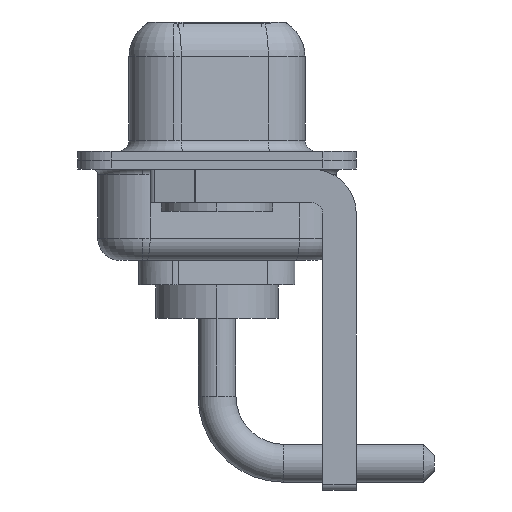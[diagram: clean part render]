
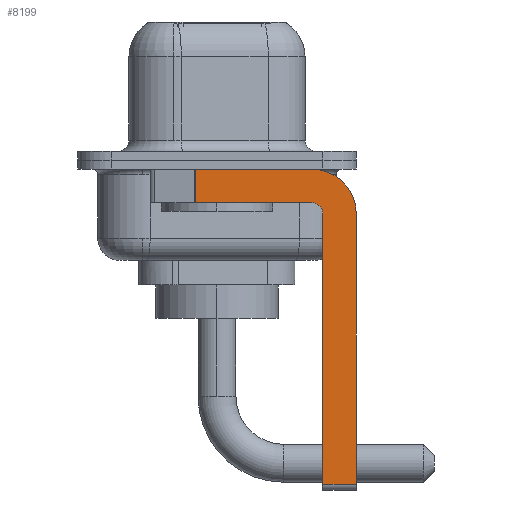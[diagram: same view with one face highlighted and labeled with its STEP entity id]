
A CAD part, left-side view. The second image highlights one B-rep face of the part: STEP entity #8199.
In plain terms, the highlighted planar face has unit normal (-1, 0, 0).
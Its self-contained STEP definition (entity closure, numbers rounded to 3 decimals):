
#23 = CARTESIAN_POINT ( 'NONE',  ( -2.9, -4.25, -2.4 ) ) ;
#88 = EDGE_CURVE ( 'NONE', #8358, #3053, #6449, .T. ) ;
#173 = VECTOR ( 'NONE', #2546, 1000. ) ;
#366 = AXIS2_PLACEMENT_3D ( 'NONE', #23, #11373, #2011 ) ;
#409 = CIRCLE ( 'NONE', #2136, 2. ) ;
#891 = CARTESIAN_POINT ( 'NONE',  ( -2.9, -4.25, -1.9 ) ) ;
#1414 = ORIENTED_EDGE ( 'NONE', *, *, #10089, .F. ) ;
#1885 = PLANE ( 'NONE',  #10585 ) ;
#2011 = DIRECTION ( 'NONE',  ( 0., 0., 1. ) ) ;
#2014 = DIRECTION ( 'NONE',  ( 0., 0., -1. ) ) ;
#2136 = AXIS2_PLACEMENT_3D ( 'NONE', #3379, #11724, #5716 ) ;
#2546 = DIRECTION ( 'NONE',  ( 0., 0., 1. ) ) ;
#2750 = VECTOR ( 'NONE', #5002, 1000. ) ;
#3053 = VERTEX_POINT ( 'NONE', #6929 ) ;
#3113 = CARTESIAN_POINT ( 'NONE',  ( -2.9, 0.978, -1.9 ) ) ;
#3173 = EDGE_CURVE ( 'NONE', #9849, #12831, #9085, .T. ) ;
#3239 = CARTESIAN_POINT ( 'NONE',  ( -2.9, -4.75, -14.55 ) ) ;
#3241 = CARTESIAN_POINT ( 'NONE',  ( -2.9, -4.75, -2.4 ) ) ;
#3379 = CARTESIAN_POINT ( 'NONE',  ( -2.9, -4.25, -2.4 ) ) ;
#3424 = EDGE_CURVE ( 'NONE', #8645, #9142, #409, .T. ) ;
#3811 = VECTOR ( 'NONE', #5895, 1000. ) ;
#4056 = EDGE_CURVE ( 'NONE', #10134, #8645, #8183, .T. ) ;
#4769 = DIRECTION ( 'NONE',  ( 0., 1., 0. ) ) ;
#4786 = EDGE_CURVE ( 'NONE', #12831, #7697, #13028, .T. ) ;
#4844 = ORIENTED_EDGE ( 'NONE', *, *, #5857, .T. ) ;
#5002 = DIRECTION ( 'NONE',  ( 0., -1., 0. ) ) ;
#5039 = FACE_OUTER_BOUND ( 'NONE', #12159, .T. ) ;
#5440 = DIRECTION ( 'NONE',  ( 0., -1., 0. ) ) ;
#5539 = ORIENTED_EDGE ( 'NONE', *, *, #88, .T. ) ;
#5698 = LINE ( 'NONE', #9858, #3811 ) ;
#5716 = DIRECTION ( 'NONE',  ( 0., 0., -1. ) ) ;
#5857 = EDGE_CURVE ( 'NONE', #10134, #7697, #5698, .T. ) ;
#5867 = ORIENTED_EDGE ( 'NONE', *, *, #3173, .F. ) ;
#5895 = DIRECTION ( 'NONE',  ( 0., 0., -1. ) ) ;
#6449 = LINE ( 'NONE', #10602, #9518 ) ;
#6718 = ORIENTED_EDGE ( 'NONE', *, *, #4056, .F. ) ;
#6838 = VECTOR ( 'NONE', #4769, 1000. ) ;
#6929 = CARTESIAN_POINT ( 'NONE',  ( -2.9, -6.25, -14.55 ) ) ;
#7091 = CARTESIAN_POINT ( 'NONE',  ( -2.9, -4.25, -0.4 ) ) ;
#7697 = VERTEX_POINT ( 'NONE', #3113 ) ;
#7722 = LINE ( 'NONE', #8682, #173 ) ;
#8183 = LINE ( 'NONE', #12566, #2750 ) ;
#8199 = ADVANCED_FACE ( 'NONE', ( #5039 ), #1885, .F. ) ;
#8358 = VERTEX_POINT ( 'NONE', #3239 ) ;
#8629 = ORIENTED_EDGE ( 'NONE', *, *, #12479, .F. ) ;
#8645 = VERTEX_POINT ( 'NONE', #7091 ) ;
#8682 = CARTESIAN_POINT ( 'NONE',  ( -2.9, -4.75, -14.8 ) ) ;
#9085 = CIRCLE ( 'NONE', #366, 0.5 ) ;
#9142 = VERTEX_POINT ( 'NONE', #11463 ) ;
#9175 = ORIENTED_EDGE ( 'NONE', *, *, #4786, .F. ) ;
#9313 = DIRECTION ( 'NONE',  ( 1., 0., 0. ) ) ;
#9513 = LINE ( 'NONE', #12799, #11498 ) ;
#9518 = VECTOR ( 'NONE', #5440, 1000. ) ;
#9827 = CARTESIAN_POINT ( 'NONE',  ( -2.9, -4.25, -1.9 ) ) ;
#9849 = VERTEX_POINT ( 'NONE', #3241 ) ;
#9858 = CARTESIAN_POINT ( 'NONE',  ( -2.9, 0.978, -1.9 ) ) ;
#10089 = EDGE_CURVE ( 'NONE', #9142, #3053, #9513, .T. ) ;
#10134 = VERTEX_POINT ( 'NONE', #11785 ) ;
#10585 = AXIS2_PLACEMENT_3D ( 'NONE', #12336, #9313, #2014 ) ;
#10602 = CARTESIAN_POINT ( 'NONE',  ( -2.9, -4.25, -14.55 ) ) ;
#10842 = ORIENTED_EDGE ( 'NONE', *, *, #3424, .F. ) ;
#11373 = DIRECTION ( 'NONE',  ( -1., 0., 0. ) ) ;
#11463 = CARTESIAN_POINT ( 'NONE',  ( -2.9, -6.25, -2.4 ) ) ;
#11498 = VECTOR ( 'NONE', #12582, 1000. ) ;
#11724 = DIRECTION ( 'NONE',  ( 1., 0., 0. ) ) ;
#11785 = CARTESIAN_POINT ( 'NONE',  ( -2.9, 0.978, -0.4 ) ) ;
#12159 = EDGE_LOOP ( 'NONE', ( #6718, #4844, #9175, #5867, #8629, #5539, #1414, #10842 ) ) ;
#12336 = CARTESIAN_POINT ( 'NONE',  ( -2.9, -4.25, -2.4 ) ) ;
#12479 = EDGE_CURVE ( 'NONE', #8358, #9849, #7722, .T. ) ;
#12566 = CARTESIAN_POINT ( 'NONE',  ( -2.9, 3., -0.4 ) ) ;
#12582 = DIRECTION ( 'NONE',  ( 0., 0., -1. ) ) ;
#12799 = CARTESIAN_POINT ( 'NONE',  ( -2.9, -6.25, -2.4 ) ) ;
#12831 = VERTEX_POINT ( 'NONE', #891 ) ;
#13028 = LINE ( 'NONE', #9827, #6838 ) ;
